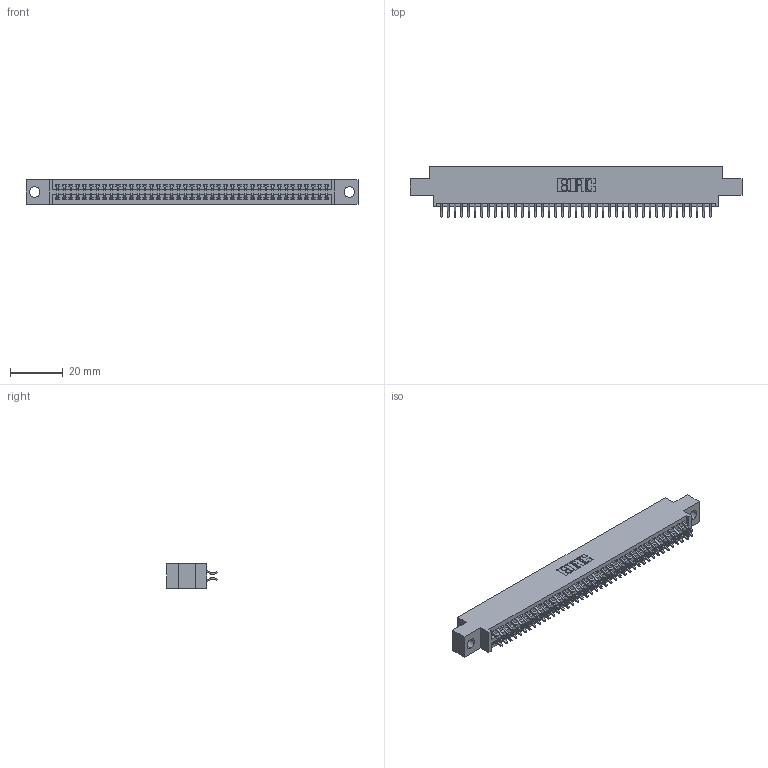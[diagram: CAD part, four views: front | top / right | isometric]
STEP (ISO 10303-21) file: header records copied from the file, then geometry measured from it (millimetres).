
FILE_DESCRIPTION (( 'STEP AP203' ), '1' );
FILE_NAME ('345-082-556-804.STEP', '2018-10-03T23:16:53', ( '' ), ( '' ), 'SwSTEP 2.0', 'SolidWorks 2016', '' );
FILE_SCHEMA (( 'CONFIG_CONTROL_DESIGN' ));
Length unit declared in the file: inch
Products named in the file (3): 345 Part_0.170 Offset - 0.156 Dia-TH; 345-292-001_556 Tail; 345-082-556-804
Assembly tree (83 placements, depth 2):
  345-082-556-804
    345 Part_0.170 Offset - 0.156 Dia-TH
    345-292-001_556 Tail  x82
Bounding box: 125.35 x 19.24 x 9.4 mm (x, y, z)
Volume: 11962.8 mm3; surface area: 17550.5 mm2
Topology: 83 solids, 83 shells, 4722 faces, 14047 edges, 9254 vertices
Faces by surface type: plane 3118, cylinder 1604
Entity records: 32659 total; most frequent: CARTESIAN_POINT 5492, ORIENTED_EDGE 5414, DIRECTION 4831, EDGE_CURVE 2707, VECTOR 2403, LINE 2403, VERTEX_POINT 1802, AXIS2_PLACEMENT_3D 1214
